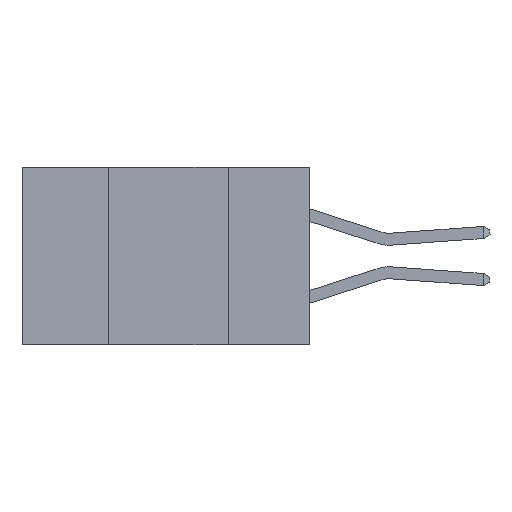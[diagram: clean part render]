
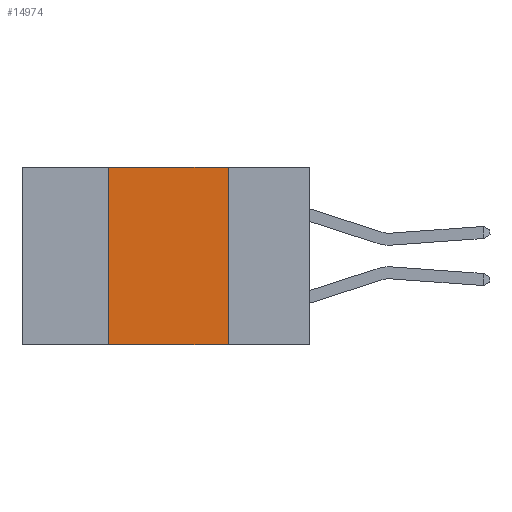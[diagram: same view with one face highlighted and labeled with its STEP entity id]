
A CAD part, left-side view. The second image highlights one B-rep face of the part: STEP entity #14974.
In plain terms, the highlighted planar face has unit normal (-1, 0, 0).
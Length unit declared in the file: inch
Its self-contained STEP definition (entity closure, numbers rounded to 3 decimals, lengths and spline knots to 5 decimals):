
#168 = EDGE_CURVE ( 'NONE', #12077, #1925, #12536, .T. ) ;
#234 = ORIENTED_EDGE ( 'NONE', *, *, #13170, .F. ) ;
#325 = LINE ( 'NONE', #4677, #12559 ) ;
#1794 = AXIS2_PLACEMENT_3D ( 'NONE', #15194, #4571, #12848 ) ;
#1925 = VERTEX_POINT ( 'NONE', #11381 ) ;
#2179 = DIRECTION ( 'NONE',  ( 0., -1., 0. ) ) ;
#3980 = CARTESIAN_POINT ( 'NONE',  ( 0., 0.42, 0. ) ) ;
#4128 = CARTESIAN_POINT ( 'NONE',  ( 0., 0.6, 0. ) ) ;
#4431 = EDGE_CURVE ( 'NONE', #11234, #12077, #10436, .T. ) ;
#4571 = DIRECTION ( 'NONE',  ( 1., 0., 0. ) ) ;
#4677 = CARTESIAN_POINT ( 'NONE',  ( 0., 0.6, -0.37 ) ) ;
#5649 = ORIENTED_EDGE ( 'NONE', *, *, #4431, .F. ) ;
#5997 = ORIENTED_EDGE ( 'NONE', *, *, #168, .F. ) ;
#6258 = VECTOR ( 'NONE', #12890, 39.37008 ) ;
#6714 = EDGE_LOOP ( 'NONE', ( #5997, #5649, #234, #13578 ) ) ;
#7391 = CARTESIAN_POINT ( 'NONE',  ( 0., 0.42, -0.37 ) ) ;
#8034 = VECTOR ( 'NONE', #2179, 39.37008 ) ;
#8273 = LINE ( 'NONE', #3980, #11792 ) ;
#8405 = EDGE_CURVE ( 'NONE', #9881, #1925, #325, .T. ) ;
#9873 = CARTESIAN_POINT ( 'NONE',  ( 0., 0.42, 0. ) ) ;
#9881 = VERTEX_POINT ( 'NONE', #7391 ) ;
#10436 = LINE ( 'NONE', #4128, #8034 ) ;
#11234 = VERTEX_POINT ( 'NONE', #9873 ) ;
#11381 = CARTESIAN_POINT ( 'NONE',  ( 0., 0.17, -0.37 ) ) ;
#11644 = PLANE ( 'NONE',  #1794 ) ;
#11792 = VECTOR ( 'NONE', #12256, 39.37008 ) ;
#12077 = VERTEX_POINT ( 'NONE', #14930 ) ;
#12256 = DIRECTION ( 'NONE',  ( 0., 0., 1. ) ) ;
#12536 = LINE ( 'NONE', #13439, #6258 ) ;
#12559 = VECTOR ( 'NONE', #14137, 39.37008 ) ;
#12848 = DIRECTION ( 'NONE',  ( 0., 0., -1. ) ) ;
#12890 = DIRECTION ( 'NONE',  ( 0., 0., -1. ) ) ;
#13170 = EDGE_CURVE ( 'NONE', #9881, #11234, #8273, .T. ) ;
#13439 = CARTESIAN_POINT ( 'NONE',  ( 0., 0.17, 0. ) ) ;
#13578 = ORIENTED_EDGE ( 'NONE', *, *, #8405, .T. ) ;
#14137 = DIRECTION ( 'NONE',  ( 0., -1., 0. ) ) ;
#14930 = CARTESIAN_POINT ( 'NONE',  ( 0., 0.17, 0. ) ) ;
#14974 = ADVANCED_FACE ( 'NONE', ( #15115 ), #11644, .F. ) ;
#15115 = FACE_OUTER_BOUND ( 'NONE', #6714, .T. ) ;
#15194 = CARTESIAN_POINT ( 'NONE',  ( 0., 0.6, 0. ) ) ;
